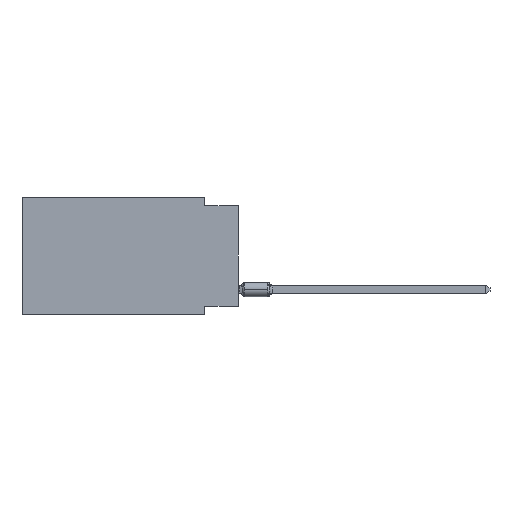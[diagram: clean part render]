
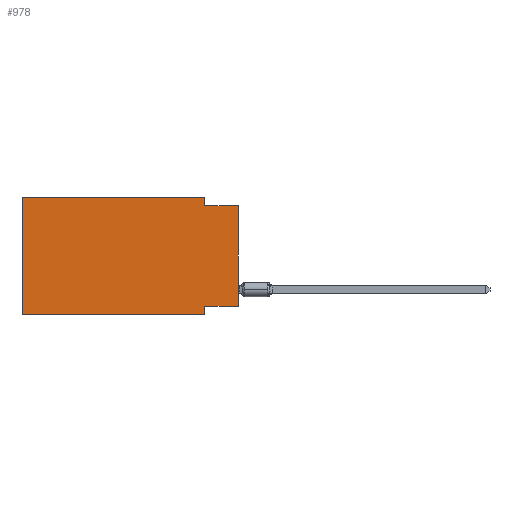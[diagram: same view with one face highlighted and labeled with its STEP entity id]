
A CAD part, left-side view. The second image highlights one B-rep face of the part: STEP entity #978.
In plain terms, the highlighted planar face has unit normal (-1, 0, 0).
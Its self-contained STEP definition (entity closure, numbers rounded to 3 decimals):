
#162 = EDGE_CURVE ( 'NONE', #4572, #9371, #2049, .T. ) ;
#254 = CARTESIAN_POINT ( 'NONE',  ( 0., 16.383, -8.89 ) ) ;
#283 = CARTESIAN_POINT ( 'NONE',  ( 0., 2.54, -8.89 ) ) ;
#475 = VERTEX_POINT ( 'NONE', #1814 ) ;
#790 = CARTESIAN_POINT ( 'NONE',  ( 0., 0., -8.255 ) ) ;
#837 = VECTOR ( 'NONE', #9540, 1000. ) ;
#978 = ADVANCED_FACE ( 'NONE', ( #2720 ), #7688, .F. ) ;
#1088 = ORIENTED_EDGE ( 'NONE', *, *, #4356, .F. ) ;
#1814 = CARTESIAN_POINT ( 'NONE',  ( 0., 2.54, 0. ) ) ;
#1929 = LINE ( 'NONE', #16596, #15259 ) ;
#2049 = LINE ( 'NONE', #8897, #20735 ) ;
#2120 = DIRECTION ( 'NONE',  ( 0., -1., 0. ) ) ;
#2282 = LINE ( 'NONE', #283, #7552 ) ;
#2469 = VECTOR ( 'NONE', #10094, 1000. ) ;
#2535 = LINE ( 'NONE', #12049, #16367 ) ;
#2599 = ORIENTED_EDGE ( 'NONE', *, *, #5048, .T. ) ;
#2720 = FACE_OUTER_BOUND ( 'NONE', #9711, .T. ) ;
#2979 = LINE ( 'NONE', #12899, #13287 ) ;
#4229 = CARTESIAN_POINT ( 'NONE',  ( 0., 2.54, -0.635 ) ) ;
#4314 = DIRECTION ( 'NONE',  ( 0., 0., -1. ) ) ;
#4356 = EDGE_CURVE ( 'NONE', #4572, #6721, #14763, .T. ) ;
#4405 = CARTESIAN_POINT ( 'NONE',  ( 0., 0., -0.635 ) ) ;
#4572 = VERTEX_POINT ( 'NONE', #790 ) ;
#5048 = EDGE_CURVE ( 'NONE', #20389, #20373, #2979, .T. ) ;
#5285 = VECTOR ( 'NONE', #10531, 1000. ) ;
#5337 = DIRECTION ( 'NONE',  ( 0., 0., -1. ) ) ;
#5861 = EDGE_CURVE ( 'NONE', #12654, #475, #11456, .T. ) ;
#6721 = VERTEX_POINT ( 'NONE', #17307 ) ;
#7552 = VECTOR ( 'NONE', #5337, 1000. ) ;
#7619 = EDGE_CURVE ( 'NONE', #18266, #9371, #1929, .T. ) ;
#7688 = PLANE ( 'NONE',  #16354 ) ;
#7852 = CARTESIAN_POINT ( 'NONE',  ( 0., 16.383, 0. ) ) ;
#7940 = DIRECTION ( 'NONE',  ( 0., -1., 0. ) ) ;
#8836 = LINE ( 'NONE', #12534, #5285 ) ;
#8897 = CARTESIAN_POINT ( 'NONE',  ( 0., 0., 0. ) ) ;
#9063 = CARTESIAN_POINT ( 'NONE',  ( 0., 16.383, 0. ) ) ;
#9371 = VERTEX_POINT ( 'NONE', #4405 ) ;
#9540 = DIRECTION ( 'NONE',  ( 0., -1., 0. ) ) ;
#9711 = EDGE_LOOP ( 'NONE', ( #15441, #20369, #16226, #19489, #18051, #2599, #19461, #1088 ) ) ;
#10094 = DIRECTION ( 'NONE',  ( 0., 1., 0. ) ) ;
#10531 = DIRECTION ( 'NONE',  ( 0., 0., 1. ) ) ;
#10545 = DIRECTION ( 'NONE',  ( 0., 0., -1. ) ) ;
#11456 = LINE ( 'NONE', #7852, #837 ) ;
#11678 = DIRECTION ( 'NONE',  ( 0., 0., 1. ) ) ;
#12049 = CARTESIAN_POINT ( 'NONE',  ( 0., 2.54, 0. ) ) ;
#12534 = CARTESIAN_POINT ( 'NONE',  ( 0., 16.383, 0. ) ) ;
#12654 = VERTEX_POINT ( 'NONE', #15702 ) ;
#12831 = EDGE_CURVE ( 'NONE', #6721, #20373, #2282, .T. ) ;
#12899 = CARTESIAN_POINT ( 'NONE',  ( 0., 16.383, -8.89 ) ) ;
#13287 = VECTOR ( 'NONE', #7940, 1000. ) ;
#13475 = CARTESIAN_POINT ( 'NONE',  ( 0., 0., -8.255 ) ) ;
#14763 = LINE ( 'NONE', #13475, #2469 ) ;
#14935 = EDGE_CURVE ( 'NONE', #475, #18266, #2535, .T. ) ;
#15259 = VECTOR ( 'NONE', #2120, 1000. ) ;
#15441 = ORIENTED_EDGE ( 'NONE', *, *, #162, .T. ) ;
#15702 = CARTESIAN_POINT ( 'NONE',  ( 0., 16.383, 0. ) ) ;
#16226 = ORIENTED_EDGE ( 'NONE', *, *, #14935, .F. ) ;
#16354 = AXIS2_PLACEMENT_3D ( 'NONE', #9063, #17106, #4314 ) ;
#16367 = VECTOR ( 'NONE', #10545, 1000. ) ;
#16596 = CARTESIAN_POINT ( 'NONE',  ( 0., 0., -0.635 ) ) ;
#17106 = DIRECTION ( 'NONE',  ( 1., 0., 0. ) ) ;
#17307 = CARTESIAN_POINT ( 'NONE',  ( 0., 2.54, -8.255 ) ) ;
#18051 = ORIENTED_EDGE ( 'NONE', *, *, #19821, .F. ) ;
#18266 = VERTEX_POINT ( 'NONE', #4229 ) ;
#19461 = ORIENTED_EDGE ( 'NONE', *, *, #12831, .F. ) ;
#19480 = CARTESIAN_POINT ( 'NONE',  ( 0., 2.54, -8.89 ) ) ;
#19489 = ORIENTED_EDGE ( 'NONE', *, *, #5861, .F. ) ;
#19821 = EDGE_CURVE ( 'NONE', #20389, #12654, #8836, .T. ) ;
#20369 = ORIENTED_EDGE ( 'NONE', *, *, #7619, .F. ) ;
#20373 = VERTEX_POINT ( 'NONE', #19480 ) ;
#20389 = VERTEX_POINT ( 'NONE', #254 ) ;
#20735 = VECTOR ( 'NONE', #11678, 1000. ) ;
